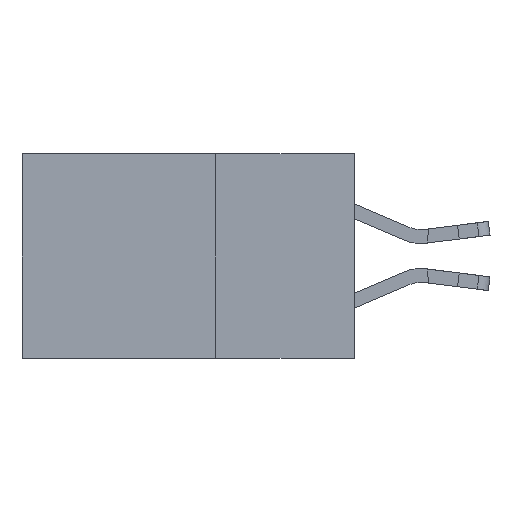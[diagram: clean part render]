
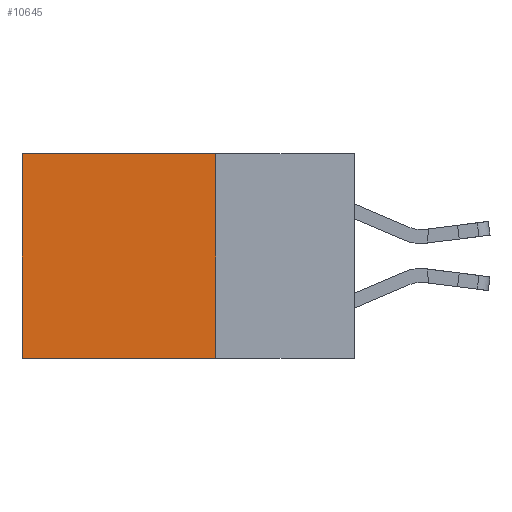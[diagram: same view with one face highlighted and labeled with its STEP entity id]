
A CAD part, left-side view. The second image highlights one B-rep face of the part: STEP entity #10645.
In plain terms, the highlighted planar face has unit normal (-1, 0, 0).
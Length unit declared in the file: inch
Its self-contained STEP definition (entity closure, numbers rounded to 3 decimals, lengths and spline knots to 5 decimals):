
#909 = DIRECTION ( 'NONE',  ( 0., 0., -1. ) ) ;
#1485 = CARTESIAN_POINT ( 'NONE',  ( 0.2615, 0.25, -0.37 ) ) ;
#1654 = EDGE_CURVE ( 'NONE', #5764, #5756, #11313, .T. ) ;
#2752 = VERTEX_POINT ( 'NONE', #10110 ) ;
#2829 = DIRECTION ( 'NONE',  ( 1., 0., 0. ) ) ;
#3415 = ORIENTED_EDGE ( 'NONE', *, *, #17287, .T. ) ;
#3886 = VECTOR ( 'NONE', #6961, 39.37008 ) ;
#3896 = ORIENTED_EDGE ( 'NONE', *, *, #1654, .F. ) ;
#4131 = CARTESIAN_POINT ( 'NONE',  ( 0.2615, 0.25, -0.37 ) ) ;
#4435 = FACE_OUTER_BOUND ( 'NONE', #17374, .T. ) ;
#4650 = CARTESIAN_POINT ( 'NONE',  ( 0.2615, 0.6, -0.37 ) ) ;
#4726 = LINE ( 'NONE', #8053, #16218 ) ;
#5631 = CARTESIAN_POINT ( 'NONE',  ( 0.2615, 0.6, 0. ) ) ;
#5756 = VERTEX_POINT ( 'NONE', #4650 ) ;
#5764 = VERTEX_POINT ( 'NONE', #12600 ) ;
#5766 = CARTESIAN_POINT ( 'NONE',  ( 0.2615, 0.25, 0. ) ) ;
#6273 = EDGE_CURVE ( 'NONE', #12585, #5756, #4726, .T. ) ;
#6838 = LINE ( 'NONE', #1485, #9963 ) ;
#6961 = DIRECTION ( 'NONE',  ( 0., 1., 0. ) ) ;
#8053 = CARTESIAN_POINT ( 'NONE',  ( 0.2615, 0.6, -0.37 ) ) ;
#8229 = AXIS2_PLACEMENT_3D ( 'NONE', #4131, #2829, #909 ) ;
#9963 = VECTOR ( 'NONE', #14594, 39.37008 ) ;
#10110 = CARTESIAN_POINT ( 'NONE',  ( 0.2615, 0.25, 0. ) ) ;
#10287 = VECTOR ( 'NONE', #14552, 39.37008 ) ;
#10492 = ORIENTED_EDGE ( 'NONE', *, *, #13203, .F. ) ;
#10645 = ADVANCED_FACE ( 'NONE', ( #4435 ), #10982, .F. ) ;
#10982 = PLANE ( 'NONE',  #8229 ) ;
#11313 = LINE ( 'NONE', #17672, #10287 ) ;
#12585 = VERTEX_POINT ( 'NONE', #5631 ) ;
#12600 = CARTESIAN_POINT ( 'NONE',  ( 0.2615, 0.25, -0.37 ) ) ;
#13203 = EDGE_CURVE ( 'NONE', #2752, #5764, #6838, .T. ) ;
#14552 = DIRECTION ( 'NONE',  ( 0., 1., 0. ) ) ;
#14594 = DIRECTION ( 'NONE',  ( 0., 0., -1. ) ) ;
#16218 = VECTOR ( 'NONE', #16342, 39.37008 ) ;
#16342 = DIRECTION ( 'NONE',  ( 0., 0., -1. ) ) ;
#16749 = LINE ( 'NONE', #5766, #3886 ) ;
#17287 = EDGE_CURVE ( 'NONE', #2752, #12585, #16749, .T. ) ;
#17374 = EDGE_LOOP ( 'NONE', ( #17406, #3896, #10492, #3415 ) ) ;
#17406 = ORIENTED_EDGE ( 'NONE', *, *, #6273, .T. ) ;
#17672 = CARTESIAN_POINT ( 'NONE',  ( 0.2615, 0.25, -0.37 ) ) ;
